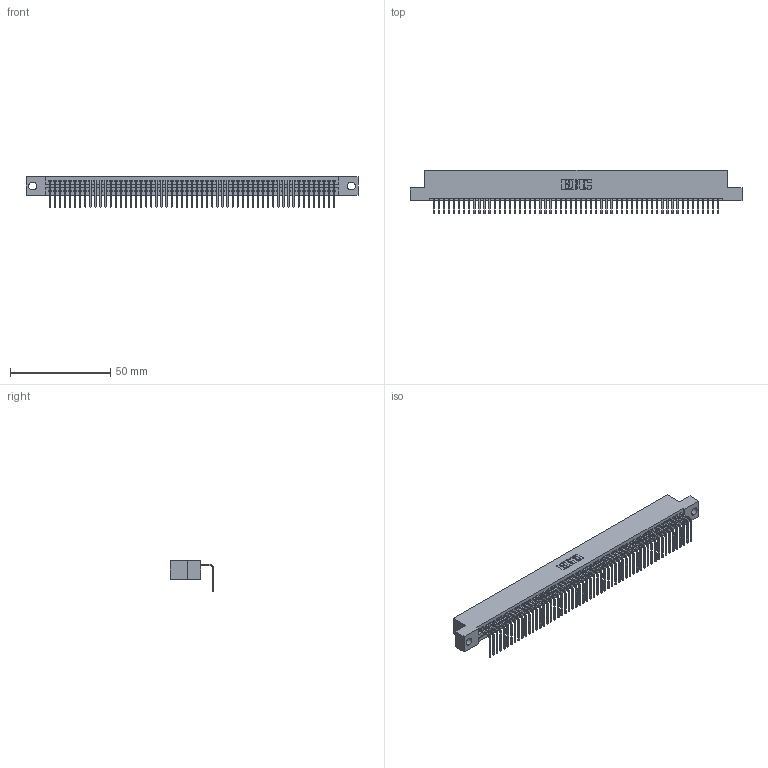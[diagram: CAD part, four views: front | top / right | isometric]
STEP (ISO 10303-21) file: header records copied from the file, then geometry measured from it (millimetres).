
FILE_DESCRIPTION (( 'STEP AP203' ), '1' );
FILE_NAME ('395-057-558-104.STEP', '2018-11-22T23:20:29', ( '' ), ( '' ), 'SwSTEP 2.0', 'SolidWorks 2016', '' );
FILE_SCHEMA (( 'CONFIG_CONTROL_DESIGN' ));
Length unit declared in the file: inch
Products named in the file (3): 395-057-558-104; 345-292-001_558 Tail - 2; 345 Part_Flush Mounting Lugs - 0.156 Dia-TH
Assembly tree (58 placements, depth 2):
  395-057-558-104
    345 Part_Flush Mounting Lugs - 0.156 Dia-TH
    345-292-001_558 Tail - 2  x57
Bounding box: 165.99 x 21.83 x 15.37 mm (x, y, z)
Volume: 15990.7 mm3; surface area: 22378.8 mm2
Topology: 58 solids, 58 shells, 3546 faces, 10715 edges, 7066 vertices
Faces by surface type: plane 2474, cylinder 1072
Entity records: 40967 total; most frequent: CARTESIAN_POINT 7103, ORIENTED_EDGE 7094, DIRECTION 6181, EDGE_CURVE 3547, LINE 3187, VECTOR 3187, VERTEX_POINT 2362, AXIS2_PLACEMENT_3D 1497
